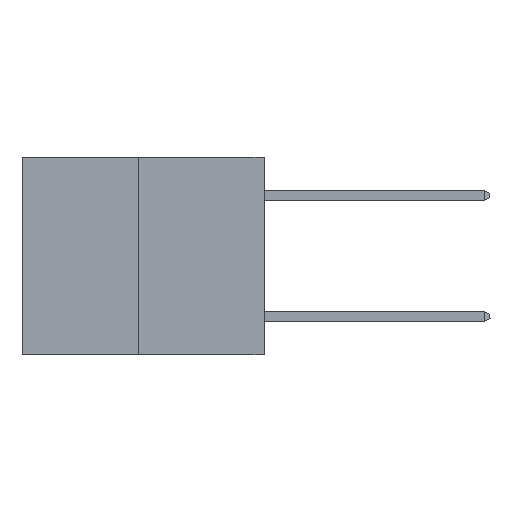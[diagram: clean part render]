
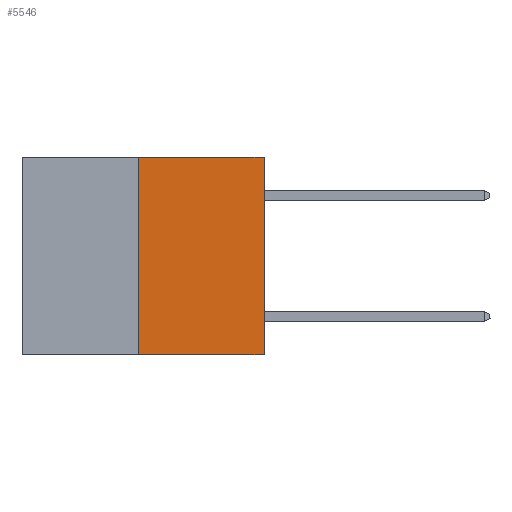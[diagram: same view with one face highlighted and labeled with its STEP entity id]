
A CAD part, left-side view. The second image highlights one B-rep face of the part: STEP entity #5546.
In plain terms, the highlighted planar face has unit normal (-1, 0, 0).
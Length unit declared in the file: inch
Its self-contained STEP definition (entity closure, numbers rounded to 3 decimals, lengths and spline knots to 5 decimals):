
#703 = VECTOR ( 'NONE', #5654, 39.37008 ) ;
#1737 = LINE ( 'NONE', #21133, #703 ) ;
#1805 = DIRECTION ( 'NONE',  ( 0., 0., 1. ) ) ;
#2045 = EDGE_CURVE ( 'NONE', #9089, #21958, #1737, .T. ) ;
#3086 = VERTEX_POINT ( 'NONE', #9953 ) ;
#3589 = EDGE_CURVE ( 'NONE', #21958, #22017, #11091, .T. ) ;
#3602 = CARTESIAN_POINT ( 'NONE',  ( 0., 0.6, 0. ) ) ;
#3818 = ORIENTED_EDGE ( 'NONE', *, *, #3589, .T. ) ;
#4361 = LINE ( 'NONE', #3602, #15307 ) ;
#4411 = EDGE_CURVE ( 'NONE', #3086, #22017, #4361, .T. ) ;
#4842 = CARTESIAN_POINT ( 'NONE',  ( 0., 0.6, 0. ) ) ;
#5546 = ADVANCED_FACE ( 'NONE', ( #12765 ), #11758, .F. ) ;
#5654 = DIRECTION ( 'NONE',  ( 0., -1., 0. ) ) ;
#5882 = AXIS2_PLACEMENT_3D ( 'NONE', #4842, #16724, #11892 ) ;
#6620 = CARTESIAN_POINT ( 'NONE',  ( 0., 0.312, -0.49 ) ) ;
#7867 = EDGE_CURVE ( 'NONE', #9089, #3086, #12417, .T. ) ;
#9089 = VERTEX_POINT ( 'NONE', #11486 ) ;
#9953 = CARTESIAN_POINT ( 'NONE',  ( 0., 0.312, 0. ) ) ;
#10696 = CARTESIAN_POINT ( 'NONE',  ( 0., 0., 0. ) ) ;
#11091 = LINE ( 'NONE', #13641, #15299 ) ;
#11486 = CARTESIAN_POINT ( 'NONE',  ( 0., 0.312, -0.49 ) ) ;
#11758 = PLANE ( 'NONE',  #5882 ) ;
#11892 = DIRECTION ( 'NONE',  ( 0., 0., -1. ) ) ;
#12417 = LINE ( 'NONE', #6620, #14258 ) ;
#12765 = FACE_OUTER_BOUND ( 'NONE', #15906, .T. ) ;
#13554 = ORIENTED_EDGE ( 'NONE', *, *, #7867, .F. ) ;
#13641 = CARTESIAN_POINT ( 'NONE',  ( 0., 0., 0. ) ) ;
#14258 = VECTOR ( 'NONE', #18793, 39.37008 ) ;
#15299 = VECTOR ( 'NONE', #1805, 39.37008 ) ;
#15307 = VECTOR ( 'NONE', #17192, 39.37008 ) ;
#15390 = ORIENTED_EDGE ( 'NONE', *, *, #4411, .F. ) ;
#15906 = EDGE_LOOP ( 'NONE', ( #13554, #16565, #3818, #15390 ) ) ;
#16565 = ORIENTED_EDGE ( 'NONE', *, *, #2045, .T. ) ;
#16724 = DIRECTION ( 'NONE',  ( 1., 0., 0. ) ) ;
#17192 = DIRECTION ( 'NONE',  ( 0., -1., 0. ) ) ;
#18793 = DIRECTION ( 'NONE',  ( 0., 0., 1. ) ) ;
#20845 = CARTESIAN_POINT ( 'NONE',  ( 0., 0., -0.49 ) ) ;
#21133 = CARTESIAN_POINT ( 'NONE',  ( 0., 0.6, -0.49 ) ) ;
#21958 = VERTEX_POINT ( 'NONE', #20845 ) ;
#22017 = VERTEX_POINT ( 'NONE', #10696 ) ;
